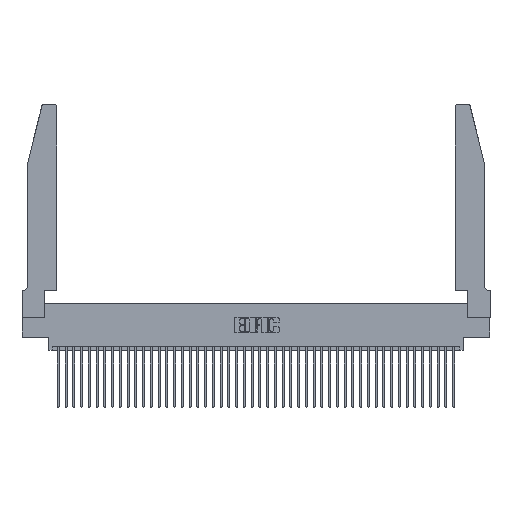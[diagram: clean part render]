
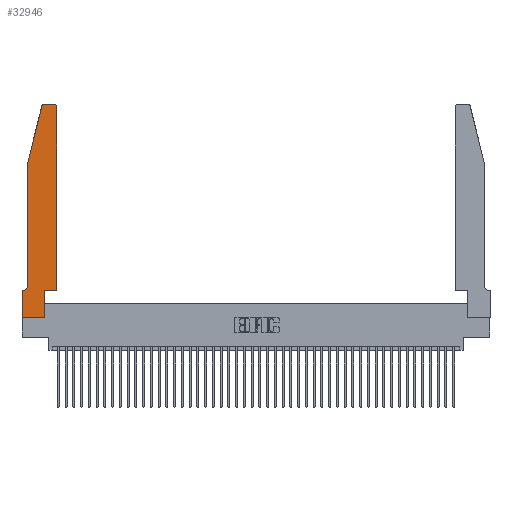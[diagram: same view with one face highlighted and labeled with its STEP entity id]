
A CAD part, top view. The second image highlights one B-rep face of the part: STEP entity #32946.
In plain terms, the highlighted planar face has unit normal (0, 0, 1).
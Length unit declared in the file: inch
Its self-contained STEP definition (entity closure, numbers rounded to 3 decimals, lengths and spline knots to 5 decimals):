
#31 = VERTEX_POINT ( 'NONE', #22349 ) ;
#723 = EDGE_CURVE ( 'NONE', #31545, #32232, #24022, .T. ) ;
#2226 = CARTESIAN_POINT ( 'NONE',  ( 0.284, 2.72, 0.37 ) ) ;
#2383 = EDGE_CURVE ( 'NONE', #12794, #34267, #23868, .T. ) ;
#2509 = EDGE_CURVE ( 'NONE', #25222, #31545, #16431, .T. ) ;
#2737 = LINE ( 'NONE', #28806, #21130 ) ;
#2901 = ORIENTED_EDGE ( 'NONE', *, *, #6245, .T. ) ;
#3347 = VERTEX_POINT ( 'NONE', #30230 ) ;
#3454 = CARTESIAN_POINT ( 'NONE',  ( 0.0755, 0.35, 0.37 ) ) ;
#3547 = CARTESIAN_POINT ( 'NONE',  ( 0., 0.35, 0.37 ) ) ;
#3932 = ORIENTED_EDGE ( 'NONE', *, *, #25447, .T. ) ;
#3999 = DIRECTION ( 'NONE',  ( 0., -1., 0. ) ) ;
#4078 = CARTESIAN_POINT ( 'NONE',  ( 0., 0.35, 0.37 ) ) ;
#4121 = AXIS2_PLACEMENT_3D ( 'NONE', #27735, #7190, #31188 ) ;
#4469 = VECTOR ( 'NONE', #3999, 39.37008 ) ;
#4592 = VECTOR ( 'NONE', #34960, 39.37008 ) ;
#4638 = CARTESIAN_POINT ( 'NONE',  ( 0.0755, 2., 0.37 ) ) ;
#4746 = CARTESIAN_POINT ( 'NONE',  ( 0.2605, 2.75, 0.37 ) ) ;
#4812 = CARTESIAN_POINT ( 'NONE',  ( 0.4205, 2.72, 0.37 ) ) ;
#5131 = DIRECTION ( 'NONE',  ( 1., 0., 0. ) ) ;
#5724 = DIRECTION ( 'NONE',  ( 1., 0., 0. ) ) ;
#6245 = EDGE_CURVE ( 'NONE', #13886, #22866, #43804, .T. ) ;
#6757 = VECTOR ( 'NONE', #5131, 39.37008 ) ;
#7074 = CARTESIAN_POINT ( 'NONE',  ( 0.4205, 2.75, 0.37 ) ) ;
#7190 = DIRECTION ( 'NONE',  ( 0., 0., -1. ) ) ;
#7429 = VECTOR ( 'NONE', #32253, 39.37008 ) ;
#8270 = CARTESIAN_POINT ( 'NONE',  ( 0.4505, 0.35, 0.37 ) ) ;
#8290 = DIRECTION ( 'NONE',  ( 1., 0., 0. ) ) ;
#8813 = CIRCLE ( 'NONE', #4121, 0.07 ) ;
#9355 = CARTESIAN_POINT ( 'NONE',  ( 0.0755, 2., 0.37 ) ) ;
#10595 = EDGE_CURVE ( 'NONE', #3347, #26977, #14904, .T. ) ;
#10966 = PLANE ( 'NONE',  #26248 ) ;
#11440 = EDGE_CURVE ( 'NONE', #34267, #31, #8813, .T. ) ;
#11771 = DIRECTION ( 'NONE',  ( -0.239, -0.971, 0. ) ) ;
#12794 = VERTEX_POINT ( 'NONE', #4638 ) ;
#13256 = VECTOR ( 'NONE', #40900, 39.37008 ) ;
#13886 = VERTEX_POINT ( 'NONE', #18079 ) ;
#13971 = ORIENTED_EDGE ( 'NONE', *, *, #723, .T. ) ;
#14356 = LINE ( 'NONE', #3454, #13256 ) ;
#14553 = CARTESIAN_POINT ( 'NONE',  ( 0.2865, 0.35, 0.37 ) ) ;
#14904 = LINE ( 'NONE', #35992, #6757 ) ;
#15419 = CARTESIAN_POINT ( 'NONE',  ( 0.0755, 0.42, 0.37 ) ) ;
#16431 = LINE ( 'NONE', #4746, #43528 ) ;
#16808 = EDGE_CURVE ( 'NONE', #26977, #13886, #22920, .T. ) ;
#17799 = CARTESIAN_POINT ( 'NONE',  ( 0.25487, 2.72718, 0.37 ) ) ;
#18065 = DIRECTION ( 'NONE',  ( 0., 0., 1. ) ) ;
#18079 = CARTESIAN_POINT ( 'NONE',  ( 0.2865, 0.35, 0.37 ) ) ;
#18308 = VECTOR ( 'NONE', #39874, 39.37008 ) ;
#20408 = VERTEX_POINT ( 'NONE', #3547 ) ;
#20567 = CARTESIAN_POINT ( 'NONE',  ( 0.4505, 0.35, 0.37 ) ) ;
#20973 = ORIENTED_EDGE ( 'NONE', *, *, #39577, .T. ) ;
#21130 = VECTOR ( 'NONE', #11771, 39.37008 ) ;
#22349 = CARTESIAN_POINT ( 'NONE',  ( 0.0055, 0.35, 0.37 ) ) ;
#22866 = VERTEX_POINT ( 'NONE', #40809 ) ;
#22920 = LINE ( 'NONE', #14553, #4592 ) ;
#23029 = LINE ( 'NONE', #20567, #40070 ) ;
#23868 = LINE ( 'NONE', #9355, #4469 ) ;
#23957 = DIRECTION ( 'NONE',  ( 0., 1., 0. ) ) ;
#24022 = CIRCLE ( 'NONE', #40569, 0.03 ) ;
#24520 = CARTESIAN_POINT ( 'NONE',  ( 0.284, 2.75, 0.37 ) ) ;
#25222 = VERTEX_POINT ( 'NONE', #7074 ) ;
#25447 = EDGE_CURVE ( 'NONE', #32232, #12794, #2737, .T. ) ;
#26248 = AXIS2_PLACEMENT_3D ( 'NONE', #4078, #18065, #41815 ) ;
#26302 = DIRECTION ( 'NONE',  ( 0., 0., 1. ) ) ;
#26977 = VERTEX_POINT ( 'NONE', #27053 ) ;
#27053 = CARTESIAN_POINT ( 'NONE',  ( 0.2865, 0., 0.37 ) ) ;
#27327 = LINE ( 'NONE', #39722, #18308 ) ;
#27735 = CARTESIAN_POINT ( 'NONE',  ( 0.0055, 0.42, 0.37 ) ) ;
#28786 = DIRECTION ( 'NONE',  ( -1., 0., 0. ) ) ;
#28806 = CARTESIAN_POINT ( 'NONE',  ( 0.0755, 2., 0.37 ) ) ;
#28840 = DIRECTION ( 'NONE',  ( 0., 0., 1. ) ) ;
#30230 = CARTESIAN_POINT ( 'NONE',  ( 0., 0., 0.37 ) ) ;
#30579 = ORIENTED_EDGE ( 'NONE', *, *, #39718, .T. ) ;
#30925 = ORIENTED_EDGE ( 'NONE', *, *, #11440, .T. ) ;
#31134 = ORIENTED_EDGE ( 'NONE', *, *, #2383, .T. ) ;
#31188 = DIRECTION ( 'NONE',  ( -1., 0., 0. ) ) ;
#31545 = VERTEX_POINT ( 'NONE', #24520 ) ;
#32232 = VERTEX_POINT ( 'NONE', #17799 ) ;
#32253 = DIRECTION ( 'NONE',  ( 1., 0., 0. ) ) ;
#32897 = ORIENTED_EDGE ( 'NONE', *, *, #2509, .T. ) ;
#32946 = ADVANCED_FACE ( 'NONE', ( #34119 ), #10966, .T. ) ;
#33516 = ORIENTED_EDGE ( 'NONE', *, *, #33571, .T. ) ;
#33571 = EDGE_CURVE ( 'NONE', #36012, #25222, #40273, .T. ) ;
#34119 = FACE_OUTER_BOUND ( 'NONE', #37210, .T. ) ;
#34267 = VERTEX_POINT ( 'NONE', #15419 ) ;
#34960 = DIRECTION ( 'NONE',  ( 0., 1., 0. ) ) ;
#35992 = CARTESIAN_POINT ( 'NONE',  ( 0., 0., 0.37 ) ) ;
#36012 = VERTEX_POINT ( 'NONE', #42814 ) ;
#37210 = EDGE_LOOP ( 'NONE', ( #32897, #13971, #3932, #31134, #30925, #39630, #20973, #37800, #37336, #2901, #30579, #33516 ) ) ;
#37336 = ORIENTED_EDGE ( 'NONE', *, *, #16808, .T. ) ;
#37800 = ORIENTED_EDGE ( 'NONE', *, *, #10595, .T. ) ;
#39577 = EDGE_CURVE ( 'NONE', #20408, #3347, #27327, .T. ) ;
#39630 = ORIENTED_EDGE ( 'NONE', *, *, #42514, .T. ) ;
#39718 = EDGE_CURVE ( 'NONE', #22866, #36012, #23029, .T. ) ;
#39722 = CARTESIAN_POINT ( 'NONE',  ( 0., 0., 0.37 ) ) ;
#39874 = DIRECTION ( 'NONE',  ( 0., -1., 0. ) ) ;
#40070 = VECTOR ( 'NONE', #23957, 39.37008 ) ;
#40273 = CIRCLE ( 'NONE', #41379, 0.03 ) ;
#40569 = AXIS2_PLACEMENT_3D ( 'NONE', #2226, #26302, #5724 ) ;
#40809 = CARTESIAN_POINT ( 'NONE',  ( 0.4505, 0.35, 0.37 ) ) ;
#40900 = DIRECTION ( 'NONE',  ( -1., 0., 0. ) ) ;
#41379 = AXIS2_PLACEMENT_3D ( 'NONE', #4812, #28840, #8290 ) ;
#41815 = DIRECTION ( 'NONE',  ( 1., 0., 0. ) ) ;
#42514 = EDGE_CURVE ( 'NONE', #31, #20408, #14356, .T. ) ;
#42814 = CARTESIAN_POINT ( 'NONE',  ( 0.4505, 2.72, 0.37 ) ) ;
#43528 = VECTOR ( 'NONE', #28786, 39.37008 ) ;
#43804 = LINE ( 'NONE', #8270, #7429 ) ;
